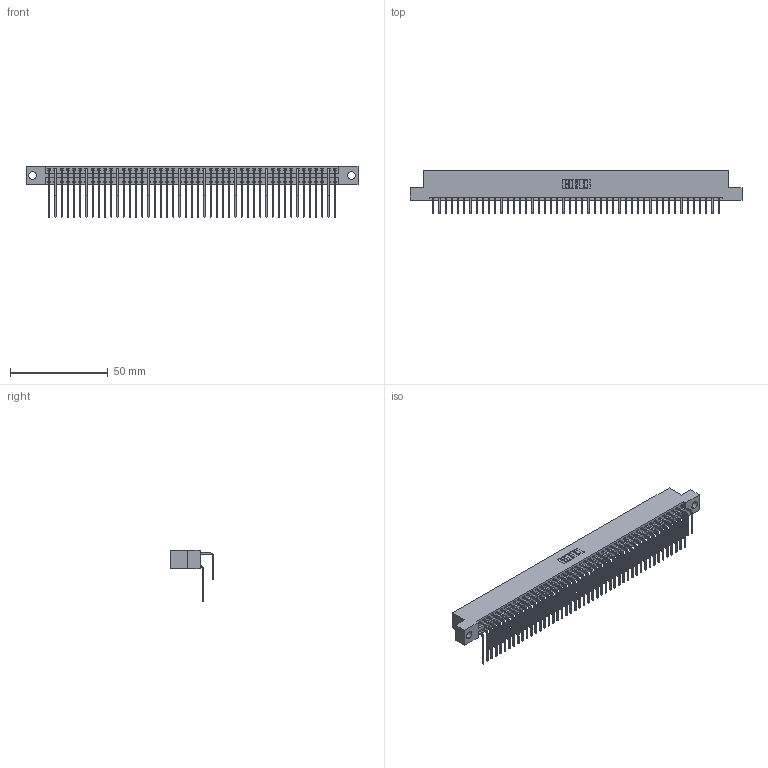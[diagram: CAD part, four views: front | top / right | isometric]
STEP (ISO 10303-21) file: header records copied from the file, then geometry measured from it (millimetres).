
FILE_DESCRIPTION (( 'STEP AP203' ), '1' );
FILE_NAME ('346-094-558-204.STEP', '2022-05-26T15:09:07', ( '' ), ( '' ), 'SwSTEP 2.0', 'SolidWorks 2020', '' );
FILE_SCHEMA (( 'CONFIG_CONTROL_DESIGN' ));
Length unit declared in the file: inch
Products named in the file (4): 345-292-001_558 559 Tail - 1; 345-292-001_558 Tail - 2; 346-094-558-204; 346 Part_Flush Mounting Lugs - 0.156 Dia-TH
Assembly tree (95 placements, depth 2):
  346-094-558-204
    346 Part_Flush Mounting Lugs - 0.156 Dia-TH
    345-292-001_558 559 Tail - 1  x47
    345-292-001_558 Tail - 2  x47
Bounding box: 169.8 x 22.16 x 26.16 mm (x, y, z)
Volume: 17032.7 mm3; surface area: 25940.4 mm2
Topology: 95 solids, 95 shells, 5212 faces, 15499 edges, 10206 vertices
Faces by surface type: plane 3568, cylinder 1644
Entity records: 32203 total; most frequent: CARTESIAN_POINT 5357, ORIENTED_EDGE 5238, DIRECTION 4743, EDGE_CURVE 2619, LINE 2259, VECTOR 2259, VERTEX_POINT 1742, AXIS2_PLACEMENT_3D 1242
